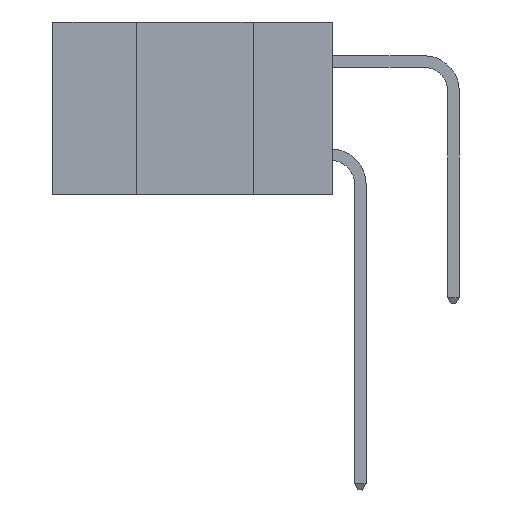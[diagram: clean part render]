
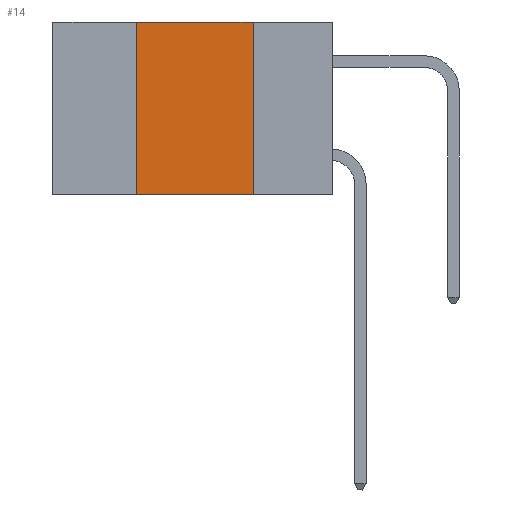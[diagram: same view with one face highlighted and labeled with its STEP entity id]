
A CAD part, left-side view. The second image highlights one B-rep face of the part: STEP entity #14.
In plain terms, the highlighted planar face has unit normal (-1, 0, 0).
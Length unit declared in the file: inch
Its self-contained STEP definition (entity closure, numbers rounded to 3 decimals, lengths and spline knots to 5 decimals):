
#14 = ADVANCED_FACE ( 'NONE', ( #11609 ), #7686, .F. ) ;
#144 = ORIENTED_EDGE ( 'NONE', *, *, #5643, .F. ) ;
#284 = EDGE_CURVE ( 'NONE', #10984, #5196, #7230, .T. ) ;
#509 = LINE ( 'NONE', #4343, #2822 ) ;
#1622 = CARTESIAN_POINT ( 'NONE',  ( 0., 0.42, 0. ) ) ;
#1688 = ORIENTED_EDGE ( 'NONE', *, *, #5913, .T. ) ;
#1712 = LINE ( 'NONE', #6522, #10957 ) ;
#2199 = ORIENTED_EDGE ( 'NONE', *, *, #9340, .F. ) ;
#2444 = VERTEX_POINT ( 'NONE', #8860 ) ;
#2822 = VECTOR ( 'NONE', #9245, 39.37008 ) ;
#2975 = CARTESIAN_POINT ( 'NONE',  ( 0., 0.17, -0.37 ) ) ;
#3220 = LINE ( 'NONE', #2975, #5243 ) ;
#4343 = CARTESIAN_POINT ( 'NONE',  ( 0., 0.6, -0.37 ) ) ;
#4862 = DIRECTION ( 'NONE',  ( 0., 0., -1. ) ) ;
#5196 = VERTEX_POINT ( 'NONE', #9646 ) ;
#5243 = VECTOR ( 'NONE', #4862, 39.37008 ) ;
#5643 = EDGE_CURVE ( 'NONE', #5196, #2444, #3220, .T. ) ;
#5913 = EDGE_CURVE ( 'NONE', #10506, #2444, #509, .T. ) ;
#6447 = DIRECTION ( 'NONE',  ( 0., -1., 0. ) ) ;
#6522 = CARTESIAN_POINT ( 'NONE',  ( 0., 0.42, -0.37 ) ) ;
#6727 = DIRECTION ( 'NONE',  ( 1., 0., 0. ) ) ;
#7227 = EDGE_LOOP ( 'NONE', ( #144, #10538, #2199, #1688 ) ) ;
#7230 = LINE ( 'NONE', #8249, #8602 ) ;
#7598 = AXIS2_PLACEMENT_3D ( 'NONE', #11540, #6727, #10595 ) ;
#7686 = PLANE ( 'NONE',  #7598 ) ;
#8249 = CARTESIAN_POINT ( 'NONE',  ( 0., 0.6, 0. ) ) ;
#8602 = VECTOR ( 'NONE', #6447, 39.37008 ) ;
#8860 = CARTESIAN_POINT ( 'NONE',  ( 0., 0.17, -0.37 ) ) ;
#8966 = CARTESIAN_POINT ( 'NONE',  ( 0., 0.42, -0.37 ) ) ;
#9245 = DIRECTION ( 'NONE',  ( 0., -1., 0. ) ) ;
#9340 = EDGE_CURVE ( 'NONE', #10506, #10984, #1712, .T. ) ;
#9646 = CARTESIAN_POINT ( 'NONE',  ( 0., 0.17, 0. ) ) ;
#10506 = VERTEX_POINT ( 'NONE', #8966 ) ;
#10538 = ORIENTED_EDGE ( 'NONE', *, *, #284, .F. ) ;
#10595 = DIRECTION ( 'NONE',  ( 0., 0., -1. ) ) ;
#10957 = VECTOR ( 'NONE', #11221, 39.37008 ) ;
#10984 = VERTEX_POINT ( 'NONE', #1622 ) ;
#11221 = DIRECTION ( 'NONE',  ( 0., 0., 1. ) ) ;
#11540 = CARTESIAN_POINT ( 'NONE',  ( 0., 0.6, 0. ) ) ;
#11609 = FACE_OUTER_BOUND ( 'NONE', #7227, .T. ) ;
